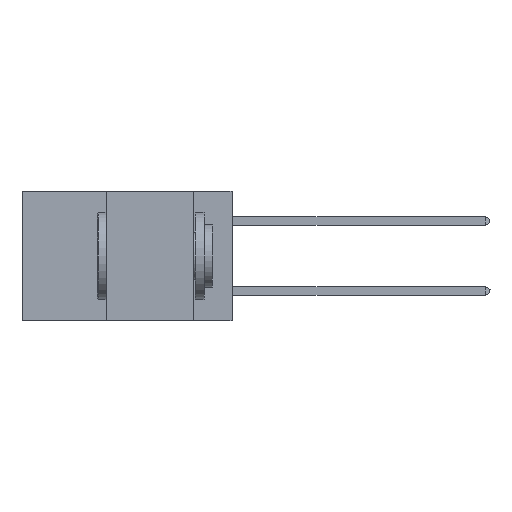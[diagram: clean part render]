
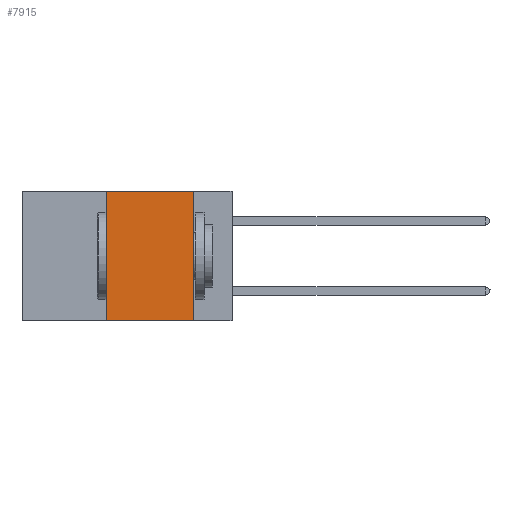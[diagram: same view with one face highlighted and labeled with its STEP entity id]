
A CAD part, left-side view. The second image highlights one B-rep face of the part: STEP entity #7915.
In plain terms, the highlighted planar face has unit normal (-1, 0, 0).
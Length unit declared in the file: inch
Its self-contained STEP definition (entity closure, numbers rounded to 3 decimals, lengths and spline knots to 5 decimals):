
#1808 = EDGE_CURVE ( 'NONE', #13441, #10163, #15838, .T. ) ;
#1940 = LINE ( 'NONE', #12718, #16579 ) ;
#3750 = VERTEX_POINT ( 'NONE', #29841 ) ;
#4418 = DIRECTION ( 'NONE',  ( 0., 0., -1. ) ) ;
#4486 = CARTESIAN_POINT ( 'NONE',  ( 0., 0.36, 0. ) ) ;
#4950 = CARTESIAN_POINT ( 'NONE',  ( 0., 0.6, -0.37 ) ) ;
#6803 = EDGE_CURVE ( 'NONE', #3750, #10163, #10335, .T. ) ;
#7915 = ADVANCED_FACE ( 'NONE', ( #24927 ), #24132, .F. ) ;
#8686 = EDGE_CURVE ( 'NONE', #3750, #23252, #17171, .T. ) ;
#9583 = DIRECTION ( 'NONE',  ( 1., 0., 0. ) ) ;
#10163 = VERTEX_POINT ( 'NONE', #10867 ) ;
#10185 = ORIENTED_EDGE ( 'NONE', *, *, #8686, .F. ) ;
#10335 = LINE ( 'NONE', #4950, #21115 ) ;
#10556 = DIRECTION ( 'NONE',  ( 0., -1., 0. ) ) ;
#10867 = CARTESIAN_POINT ( 'NONE',  ( 0., 0.11, -0.37 ) ) ;
#11948 = VECTOR ( 'NONE', #22540, 39.37008 ) ;
#12718 = CARTESIAN_POINT ( 'NONE',  ( 0., 0.6, 0. ) ) ;
#13441 = VERTEX_POINT ( 'NONE', #13785 ) ;
#13785 = CARTESIAN_POINT ( 'NONE',  ( 0., 0.11, 0. ) ) ;
#13815 = ORIENTED_EDGE ( 'NONE', *, *, #6803, .T. ) ;
#14670 = DIRECTION ( 'NONE',  ( 0., -1., 0. ) ) ;
#14929 = EDGE_CURVE ( 'NONE', #23252, #13441, #1940, .T. ) ;
#15838 = LINE ( 'NONE', #20038, #11948 ) ;
#16306 = CARTESIAN_POINT ( 'NONE',  ( 0., 0.36, 0. ) ) ;
#16579 = VECTOR ( 'NONE', #10556, 39.37008 ) ;
#17171 = LINE ( 'NONE', #4486, #19848 ) ;
#19848 = VECTOR ( 'NONE', #26674, 39.37008 ) ;
#20038 = CARTESIAN_POINT ( 'NONE',  ( 0., 0.11, 0. ) ) ;
#20713 = ORIENTED_EDGE ( 'NONE', *, *, #14929, .F. ) ;
#21115 = VECTOR ( 'NONE', #14670, 39.37008 ) ;
#21662 = EDGE_LOOP ( 'NONE', ( #30714, #20713, #10185, #13815 ) ) ;
#22540 = DIRECTION ( 'NONE',  ( 0., 0., -1. ) ) ;
#23252 = VERTEX_POINT ( 'NONE', #16306 ) ;
#24132 = PLANE ( 'NONE',  #27375 ) ;
#24348 = CARTESIAN_POINT ( 'NONE',  ( 0., 0.6, 0. ) ) ;
#24927 = FACE_OUTER_BOUND ( 'NONE', #21662, .T. ) ;
#26674 = DIRECTION ( 'NONE',  ( 0., 0., 1. ) ) ;
#27375 = AXIS2_PLACEMENT_3D ( 'NONE', #24348, #9583, #4418 ) ;
#29841 = CARTESIAN_POINT ( 'NONE',  ( 0., 0.36, -0.37 ) ) ;
#30714 = ORIENTED_EDGE ( 'NONE', *, *, #1808, .F. ) ;
